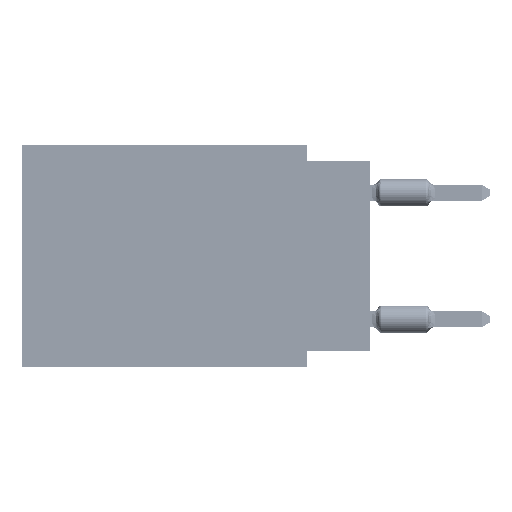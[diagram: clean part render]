
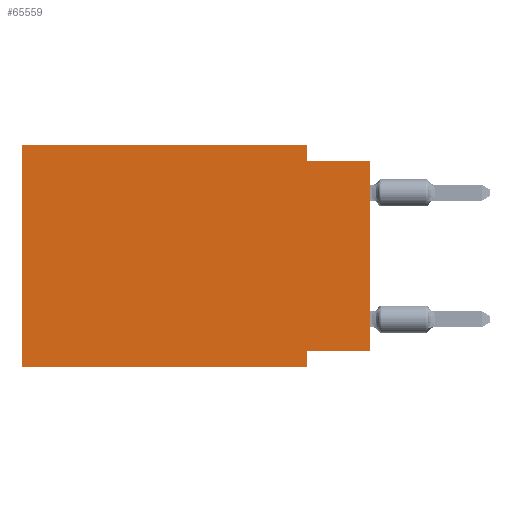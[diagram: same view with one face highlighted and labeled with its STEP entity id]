
A CAD part, left-side view. The second image highlights one B-rep face of the part: STEP entity #65559.
In plain terms, the highlighted planar face has unit normal (-1, 0, 0).
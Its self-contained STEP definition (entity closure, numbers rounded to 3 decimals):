
#689 = CARTESIAN_POINT ( 'NONE',  ( 0., 2.54, 0. ) ) ;
#1679 = CARTESIAN_POINT ( 'NONE',  ( 0., 2.54, -8.255 ) ) ;
#2084 = VERTEX_POINT ( 'NONE', #16208 ) ;
#2625 = DIRECTION ( 'NONE',  ( 0., 1., 0. ) ) ;
#3670 = LINE ( 'NONE', #46333, #24467 ) ;
#3671 = FACE_OUTER_BOUND ( 'NONE', #24363, .T. ) ;
#4028 = PLANE ( 'NONE',  #6815 ) ;
#6710 = VERTEX_POINT ( 'NONE', #1679 ) ;
#6815 = AXIS2_PLACEMENT_3D ( 'NONE', #30597, #35159, #52287 ) ;
#8848 = ORIENTED_EDGE ( 'NONE', *, *, #55778, .T. ) ;
#9254 = CARTESIAN_POINT ( 'NONE',  ( 0., 0., -8.255 ) ) ;
#10978 = EDGE_CURVE ( 'NONE', #23935, #2084, #61702, .T. ) ;
#13500 = ORIENTED_EDGE ( 'NONE', *, *, #37977, .F. ) ;
#15915 = CARTESIAN_POINT ( 'NONE',  ( 0., 0., -8.255 ) ) ;
#16052 = VECTOR ( 'NONE', #35145, 1000. ) ;
#16167 = ORIENTED_EDGE ( 'NONE', *, *, #30793, .F. ) ;
#16208 = CARTESIAN_POINT ( 'NONE',  ( 0., 0., -0.635 ) ) ;
#17657 = ORIENTED_EDGE ( 'NONE', *, *, #20393, .F. ) ;
#20274 = EDGE_CURVE ( 'NONE', #23935, #6710, #40040, .T. ) ;
#20393 = EDGE_CURVE ( 'NONE', #67723, #29712, #62443, .T. ) ;
#21810 = CARTESIAN_POINT ( 'NONE',  ( 0., 13.97, 0. ) ) ;
#23246 = CARTESIAN_POINT ( 'NONE',  ( 0., 0., 0. ) ) ;
#23935 = VERTEX_POINT ( 'NONE', #15915 ) ;
#24363 = EDGE_LOOP ( 'NONE', ( #42303, #33083, #16167, #13500, #17657, #8848, #28845, #57300 ) ) ;
#24467 = VECTOR ( 'NONE', #41089, 1000. ) ;
#28845 = ORIENTED_EDGE ( 'NONE', *, *, #59315, .F. ) ;
#29712 = VERTEX_POINT ( 'NONE', #21810 ) ;
#30101 = CARTESIAN_POINT ( 'NONE',  ( 0., 13.97, -8.89 ) ) ;
#30597 = CARTESIAN_POINT ( 'NONE',  ( 0., 13.97, 0. ) ) ;
#30793 = EDGE_CURVE ( 'NONE', #54855, #36353, #3670, .T. ) ;
#30808 = CARTESIAN_POINT ( 'NONE',  ( 0., 13.97, 0. ) ) ;
#33083 = ORIENTED_EDGE ( 'NONE', *, *, #44609, .F. ) ;
#33869 = VECTOR ( 'NONE', #2625, 1000. ) ;
#35090 = CARTESIAN_POINT ( 'NONE',  ( 0., 2.54, -0.635 ) ) ;
#35145 = DIRECTION ( 'NONE',  ( 0., 0., 1. ) ) ;
#35159 = DIRECTION ( 'NONE',  ( 1., 0., 0. ) ) ;
#36353 = VERTEX_POINT ( 'NONE', #35090 ) ;
#37977 = EDGE_CURVE ( 'NONE', #29712, #54855, #47566, .T. ) ;
#40040 = LINE ( 'NONE', #9254, #33869 ) ;
#40239 = DIRECTION ( 'NONE',  ( 0., -1., 0. ) ) ;
#41016 = VECTOR ( 'NONE', #45336, 1000. ) ;
#41089 = DIRECTION ( 'NONE',  ( 0., 0., -1. ) ) ;
#42303 = ORIENTED_EDGE ( 'NONE', *, *, #10978, .T. ) ;
#44609 = EDGE_CURVE ( 'NONE', #36353, #2084, #57636, .T. ) ;
#44770 = DIRECTION ( 'NONE',  ( 0., -1., 0. ) ) ;
#45336 = DIRECTION ( 'NONE',  ( 0., 0., -1. ) ) ;
#46333 = CARTESIAN_POINT ( 'NONE',  ( 0., 2.54, 0. ) ) ;
#47566 = LINE ( 'NONE', #30808, #62139 ) ;
#47898 = DIRECTION ( 'NONE',  ( 0., -1., 0. ) ) ;
#48375 = VECTOR ( 'NONE', #44770, 1000. ) ;
#52287 = DIRECTION ( 'NONE',  ( 0., 0., -1. ) ) ;
#54038 = VERTEX_POINT ( 'NONE', #66814 ) ;
#54855 = VERTEX_POINT ( 'NONE', #689 ) ;
#55144 = LINE ( 'NONE', #59704, #41016 ) ;
#55778 = EDGE_CURVE ( 'NONE', #67723, #54038, #61252, .T. ) ;
#56096 = CARTESIAN_POINT ( 'NONE',  ( 0., 13.97, -8.89 ) ) ;
#57300 = ORIENTED_EDGE ( 'NONE', *, *, #20274, .F. ) ;
#57636 = LINE ( 'NONE', #68443, #48375 ) ;
#59315 = EDGE_CURVE ( 'NONE', #6710, #54038, #55144, .T. ) ;
#59704 = CARTESIAN_POINT ( 'NONE',  ( 0., 2.54, -8.89 ) ) ;
#60318 = DIRECTION ( 'NONE',  ( 0., 0., 1. ) ) ;
#61252 = LINE ( 'NONE', #30101, #68788 ) ;
#61702 = LINE ( 'NONE', #23246, #61859 ) ;
#61728 = CARTESIAN_POINT ( 'NONE',  ( 0., 13.97, 0. ) ) ;
#61859 = VECTOR ( 'NONE', #60318, 1000. ) ;
#62139 = VECTOR ( 'NONE', #47898, 1000. ) ;
#62443 = LINE ( 'NONE', #61728, #16052 ) ;
#65559 = ADVANCED_FACE ( 'NONE', ( #3671 ), #4028, .F. ) ;
#66814 = CARTESIAN_POINT ( 'NONE',  ( 0., 2.54, -8.89 ) ) ;
#67723 = VERTEX_POINT ( 'NONE', #56096 ) ;
#68443 = CARTESIAN_POINT ( 'NONE',  ( 0., 0., -0.635 ) ) ;
#68788 = VECTOR ( 'NONE', #40239, 1000. ) ;
